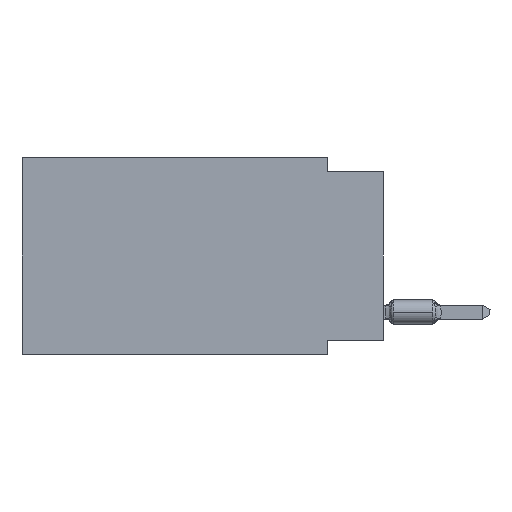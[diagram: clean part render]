
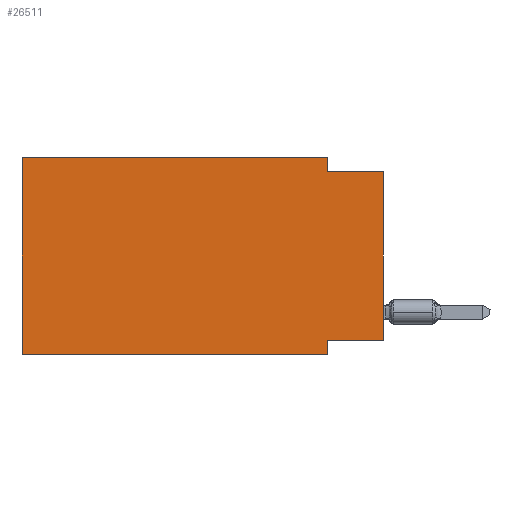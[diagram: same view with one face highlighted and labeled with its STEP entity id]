
A CAD part, left-side view. The second image highlights one B-rep face of the part: STEP entity #26511.
In plain terms, the highlighted planar face has unit normal (-1, 0, 0).
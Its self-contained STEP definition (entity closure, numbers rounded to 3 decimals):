
#29 = CARTESIAN_POINT ( 'NONE',  ( 0., 16.383, -8.89 ) ) ;
#186 = DIRECTION ( 'NONE',  ( 0., 0., -1. ) ) ;
#269 = ORIENTED_EDGE ( 'NONE', *, *, #25979, .T. ) ;
#618 = VERTEX_POINT ( 'NONE', #1026 ) ;
#849 = CARTESIAN_POINT ( 'NONE',  ( 0., 2.54, -8.255 ) ) ;
#1026 = CARTESIAN_POINT ( 'NONE',  ( 0., 0., -8.255 ) ) ;
#1469 = CARTESIAN_POINT ( 'NONE',  ( 0., 2.54, 0. ) ) ;
#2451 = EDGE_CURVE ( 'NONE', #37416, #36304, #38466, .T. ) ;
#2501 = VECTOR ( 'NONE', #31677, 1000. ) ;
#2882 = VERTEX_POINT ( 'NONE', #29110 ) ;
#3226 = PLANE ( 'NONE',  #10119 ) ;
#3603 = VECTOR ( 'NONE', #9576, 1000. ) ;
#3935 = CARTESIAN_POINT ( 'NONE',  ( 0., 16.383, -8.89 ) ) ;
#4649 = VECTOR ( 'NONE', #31492, 1000. ) ;
#4692 = DIRECTION ( 'NONE',  ( 0., 0., -1. ) ) ;
#5191 = VERTEX_POINT ( 'NONE', #12448 ) ;
#5395 = VECTOR ( 'NONE', #4692, 1000. ) ;
#5517 = EDGE_CURVE ( 'NONE', #618, #37416, #5665, .T. ) ;
#5665 = LINE ( 'NONE', #34924, #2501 ) ;
#6840 = CARTESIAN_POINT ( 'NONE',  ( 0., 16.383, 0. ) ) ;
#7046 = EDGE_CURVE ( 'NONE', #2882, #5191, #20842, .T. ) ;
#8778 = LINE ( 'NONE', #18121, #32042 ) ;
#8800 = CARTESIAN_POINT ( 'NONE',  ( 0., 2.54, -8.89 ) ) ;
#9152 = ORIENTED_EDGE ( 'NONE', *, *, #2451, .F. ) ;
#9576 = DIRECTION ( 'NONE',  ( 0., -1., 0. ) ) ;
#10119 = AXIS2_PLACEMENT_3D ( 'NONE', #16458, #23176, #186 ) ;
#12246 = CARTESIAN_POINT ( 'NONE',  ( 0., 2.54, -8.89 ) ) ;
#12448 = CARTESIAN_POINT ( 'NONE',  ( 0., 0., -0.635 ) ) ;
#12802 = ORIENTED_EDGE ( 'NONE', *, *, #39913, .F. ) ;
#14708 = VECTOR ( 'NONE', #23745, 1000. ) ;
#15150 = LINE ( 'NONE', #28371, #23546 ) ;
#16314 = EDGE_CURVE ( 'NONE', #20787, #21979, #15150, .T. ) ;
#16458 = CARTESIAN_POINT ( 'NONE',  ( 0., 16.383, 0. ) ) ;
#16605 = ORIENTED_EDGE ( 'NONE', *, *, #16314, .F. ) ;
#16681 = FACE_OUTER_BOUND ( 'NONE', #17297, .T. ) ;
#17297 = EDGE_LOOP ( 'NONE', ( #269, #39058, #12802, #22455, #16605, #42744, #9152, #42828 ) ) ;
#18121 = CARTESIAN_POINT ( 'NONE',  ( 0., 0., 0. ) ) ;
#20430 = CARTESIAN_POINT ( 'NONE',  ( 0., 16.383, 0. ) ) ;
#20787 = VERTEX_POINT ( 'NONE', #3935 ) ;
#20842 = LINE ( 'NONE', #27124, #33629 ) ;
#21753 = LINE ( 'NONE', #31701, #4649 ) ;
#21979 = VERTEX_POINT ( 'NONE', #20430 ) ;
#22455 = ORIENTED_EDGE ( 'NONE', *, *, #35432, .F. ) ;
#23176 = DIRECTION ( 'NONE',  ( 1., 0., 0. ) ) ;
#23540 = LINE ( 'NONE', #6840, #14708 ) ;
#23546 = VECTOR ( 'NONE', #31182, 1000. ) ;
#23745 = DIRECTION ( 'NONE',  ( 0., -1., 0. ) ) ;
#25464 = VERTEX_POINT ( 'NONE', #1469 ) ;
#25979 = EDGE_CURVE ( 'NONE', #618, #5191, #8778, .T. ) ;
#26275 = LINE ( 'NONE', #29, #3603 ) ;
#26511 = ADVANCED_FACE ( 'NONE', ( #16681 ), #3226, .F. ) ;
#27124 = CARTESIAN_POINT ( 'NONE',  ( 0., 0., -0.635 ) ) ;
#28371 = CARTESIAN_POINT ( 'NONE',  ( 0., 16.383, 0. ) ) ;
#29110 = CARTESIAN_POINT ( 'NONE',  ( 0., 2.54, -0.635 ) ) ;
#31182 = DIRECTION ( 'NONE',  ( 0., 0., 1. ) ) ;
#31492 = DIRECTION ( 'NONE',  ( 0., 0., -1. ) ) ;
#31533 = DIRECTION ( 'NONE',  ( 0., 0., 1. ) ) ;
#31677 = DIRECTION ( 'NONE',  ( 0., 1., 0. ) ) ;
#31701 = CARTESIAN_POINT ( 'NONE',  ( 0., 2.54, 0. ) ) ;
#32042 = VECTOR ( 'NONE', #31533, 1000. ) ;
#33614 = DIRECTION ( 'NONE',  ( 0., -1., 0. ) ) ;
#33629 = VECTOR ( 'NONE', #33614, 1000. ) ;
#34924 = CARTESIAN_POINT ( 'NONE',  ( 0., 0., -8.255 ) ) ;
#35432 = EDGE_CURVE ( 'NONE', #21979, #25464, #23540, .T. ) ;
#36304 = VERTEX_POINT ( 'NONE', #12246 ) ;
#36790 = EDGE_CURVE ( 'NONE', #20787, #36304, #26275, .T. ) ;
#37416 = VERTEX_POINT ( 'NONE', #849 ) ;
#38466 = LINE ( 'NONE', #8800, #5395 ) ;
#39058 = ORIENTED_EDGE ( 'NONE', *, *, #7046, .F. ) ;
#39913 = EDGE_CURVE ( 'NONE', #25464, #2882, #21753, .T. ) ;
#42744 = ORIENTED_EDGE ( 'NONE', *, *, #36790, .T. ) ;
#42828 = ORIENTED_EDGE ( 'NONE', *, *, #5517, .F. ) ;
